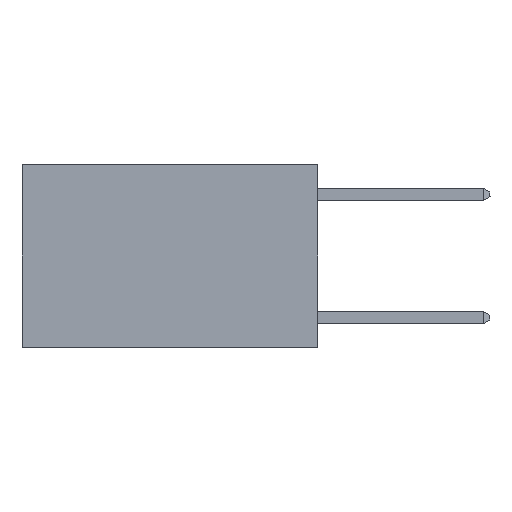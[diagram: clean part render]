
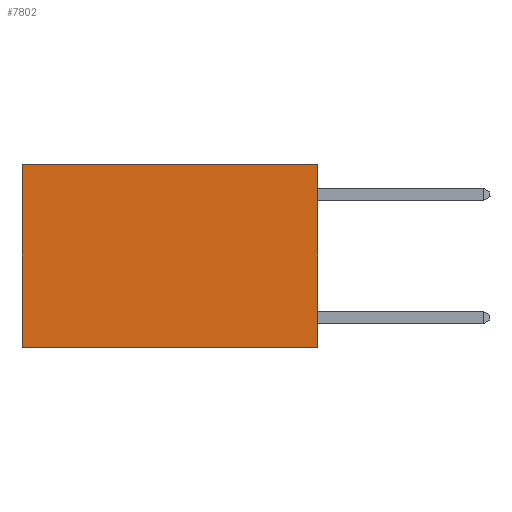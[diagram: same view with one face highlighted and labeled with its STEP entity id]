
A CAD part, left-side view. The second image highlights one B-rep face of the part: STEP entity #7802.
In plain terms, the highlighted planar face has unit normal (-1, 0, 0).
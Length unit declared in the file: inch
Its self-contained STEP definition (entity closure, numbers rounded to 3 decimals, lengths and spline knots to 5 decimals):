
#18 = VERTEX_POINT ( 'NONE', #1780 ) ;
#29 = EDGE_CURVE ( 'NONE', #7916, #2669, #6397, .T. ) ;
#395 = CARTESIAN_POINT ( 'NONE',  ( 0.2625, 0., 0. ) ) ;
#536 = CARTESIAN_POINT ( 'NONE',  ( 0.2625, 0.6, 0. ) ) ;
#573 = DIRECTION ( 'NONE',  ( 0., 0., -1. ) ) ;
#940 = PLANE ( 'NONE',  #5487 ) ;
#1299 = FACE_OUTER_BOUND ( 'NONE', #6883, .T. ) ;
#1423 = VECTOR ( 'NONE', #573, 39.37008 ) ;
#1590 = DIRECTION ( 'NONE',  ( 0., 0., -1. ) ) ;
#1748 = DIRECTION ( 'NONE',  ( 0., 1., 0. ) ) ;
#1780 = CARTESIAN_POINT ( 'NONE',  ( 0.2625, 0., -0.37 ) ) ;
#2000 = VECTOR ( 'NONE', #1748, 39.37008 ) ;
#2285 = VERTEX_POINT ( 'NONE', #6873 ) ;
#2394 = ORIENTED_EDGE ( 'NONE', *, *, #4653, .F. ) ;
#2669 = VERTEX_POINT ( 'NONE', #3472 ) ;
#2746 = CARTESIAN_POINT ( 'NONE',  ( 0.2625, 0., 0. ) ) ;
#2818 = EDGE_CURVE ( 'NONE', #2285, #18, #5156, .T. ) ;
#3439 = DIRECTION ( 'NONE',  ( 1., 0., 0. ) ) ;
#3472 = CARTESIAN_POINT ( 'NONE',  ( 0.2625, 0.6, -0.37 ) ) ;
#3519 = ORIENTED_EDGE ( 'NONE', *, *, #2818, .F. ) ;
#3988 = LINE ( 'NONE', #6267, #5235 ) ;
#4045 = LINE ( 'NONE', #4816, #2000 ) ;
#4653 = EDGE_CURVE ( 'NONE', #18, #2669, #3988, .T. ) ;
#4767 = VECTOR ( 'NONE', #5007, 39.37008 ) ;
#4816 = CARTESIAN_POINT ( 'NONE',  ( 0.2625, 0., 0. ) ) ;
#5007 = DIRECTION ( 'NONE',  ( 0., 0., -1. ) ) ;
#5156 = LINE ( 'NONE', #395, #4767 ) ;
#5235 = VECTOR ( 'NONE', #6800, 39.37008 ) ;
#5416 = EDGE_CURVE ( 'NONE', #2285, #7916, #4045, .T. ) ;
#5487 = AXIS2_PLACEMENT_3D ( 'NONE', #2746, #3439, #1590 ) ;
#6267 = CARTESIAN_POINT ( 'NONE',  ( 0.2625, 0., -0.37 ) ) ;
#6397 = LINE ( 'NONE', #6766, #1423 ) ;
#6766 = CARTESIAN_POINT ( 'NONE',  ( 0.2625, 0.6, 0. ) ) ;
#6800 = DIRECTION ( 'NONE',  ( 0., 1., 0. ) ) ;
#6873 = CARTESIAN_POINT ( 'NONE',  ( 0.2625, 0., 0. ) ) ;
#6883 = EDGE_LOOP ( 'NONE', ( #7760, #2394, #3519, #7884 ) ) ;
#7760 = ORIENTED_EDGE ( 'NONE', *, *, #29, .T. ) ;
#7802 = ADVANCED_FACE ( 'NONE', ( #1299 ), #940, .F. ) ;
#7884 = ORIENTED_EDGE ( 'NONE', *, *, #5416, .T. ) ;
#7916 = VERTEX_POINT ( 'NONE', #536 ) ;
